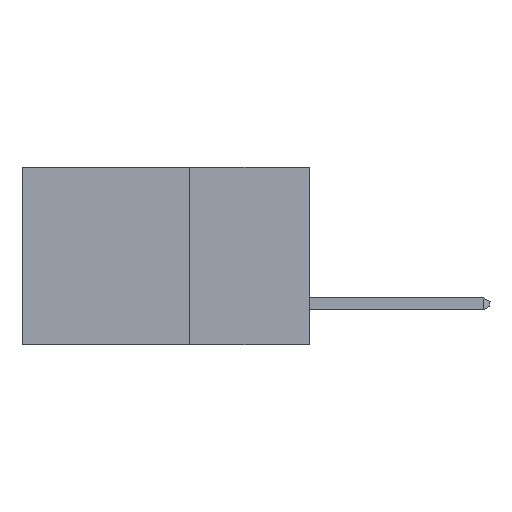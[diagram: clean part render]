
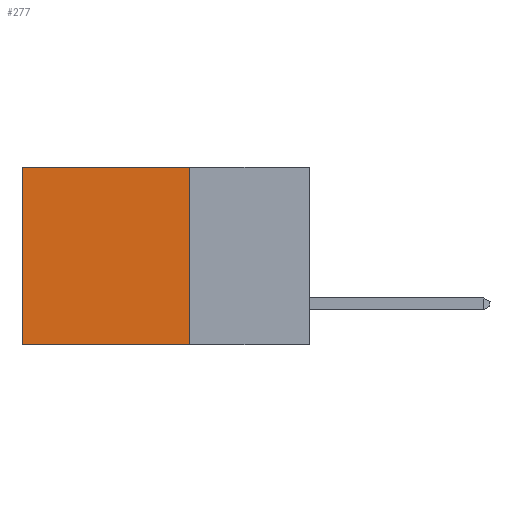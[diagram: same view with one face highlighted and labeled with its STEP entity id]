
A CAD part, left-side view. The second image highlights one B-rep face of the part: STEP entity #277.
In plain terms, the highlighted planar face has unit normal (-1, 0, 0).
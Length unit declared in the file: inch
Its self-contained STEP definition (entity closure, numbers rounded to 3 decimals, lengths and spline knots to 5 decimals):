
#158 = LINE ( 'NONE', #18844, #35405 ) ;
#277 = ADVANCED_FACE ( 'NONE', ( #43057 ), #21933, .F. ) ;
#1640 = LINE ( 'NONE', #35202, #14198 ) ;
#2919 = DIRECTION ( 'NONE',  ( 1., 0., 0. ) ) ;
#3543 = VECTOR ( 'NONE', #3761, 39.37008 ) ;
#3761 = DIRECTION ( 'NONE',  ( 0., 0., -1. ) ) ;
#5942 = LINE ( 'NONE', #11949, #3543 ) ;
#6263 = ORIENTED_EDGE ( 'NONE', *, *, #22048, .F. ) ;
#6749 = DIRECTION ( 'NONE',  ( 0., 0., -1. ) ) ;
#7228 = EDGE_CURVE ( 'NONE', #24048, #20370, #44755, .T. ) ;
#7670 = VERTEX_POINT ( 'NONE', #20473 ) ;
#9633 = DIRECTION ( 'NONE',  ( 0., 1., 0. ) ) ;
#11949 = CARTESIAN_POINT ( 'NONE',  ( 0.2875, 0.25, 0. ) ) ;
#14198 = VECTOR ( 'NONE', #9633, 39.37008 ) ;
#14347 = EDGE_CURVE ( 'NONE', #7670, #20370, #158, .T. ) ;
#17213 = VECTOR ( 'NONE', #35066, 39.37008 ) ;
#18844 = CARTESIAN_POINT ( 'NONE',  ( 0.2875, 0.6, 0. ) ) ;
#20370 = VERTEX_POINT ( 'NONE', #29235 ) ;
#20473 = CARTESIAN_POINT ( 'NONE',  ( 0.2875, 0.6, 0. ) ) ;
#21933 = PLANE ( 'NONE',  #35764 ) ;
#22048 = EDGE_CURVE ( 'NONE', #42186, #24048, #5942, .T. ) ;
#24048 = VERTEX_POINT ( 'NONE', #39874 ) ;
#24823 = ORIENTED_EDGE ( 'NONE', *, *, #7228, .F. ) ;
#25743 = CARTESIAN_POINT ( 'NONE',  ( 0.2875, 0.25, 0. ) ) ;
#29235 = CARTESIAN_POINT ( 'NONE',  ( 0.2875, 0.6, -0.37 ) ) ;
#31199 = ORIENTED_EDGE ( 'NONE', *, *, #37923, .T. ) ;
#34016 = DIRECTION ( 'NONE',  ( 0., 0., -1. ) ) ;
#35066 = DIRECTION ( 'NONE',  ( 0., 1., 0. ) ) ;
#35202 = CARTESIAN_POINT ( 'NONE',  ( 0.2875, 0.25, 0. ) ) ;
#35405 = VECTOR ( 'NONE', #34016, 39.37008 ) ;
#35628 = EDGE_LOOP ( 'NONE', ( #39053, #24823, #6263, #31199 ) ) ;
#35764 = AXIS2_PLACEMENT_3D ( 'NONE', #25743, #2919, #6749 ) ;
#37923 = EDGE_CURVE ( 'NONE', #42186, #7670, #1640, .T. ) ;
#38274 = CARTESIAN_POINT ( 'NONE',  ( 0.2875, 0.25, 0. ) ) ;
#39053 = ORIENTED_EDGE ( 'NONE', *, *, #14347, .T. ) ;
#39874 = CARTESIAN_POINT ( 'NONE',  ( 0.2875, 0.25, -0.37 ) ) ;
#42186 = VERTEX_POINT ( 'NONE', #38274 ) ;
#42643 = CARTESIAN_POINT ( 'NONE',  ( 0.2875, 0.25, -0.37 ) ) ;
#43057 = FACE_OUTER_BOUND ( 'NONE', #35628, .T. ) ;
#44755 = LINE ( 'NONE', #42643, #17213 ) ;
